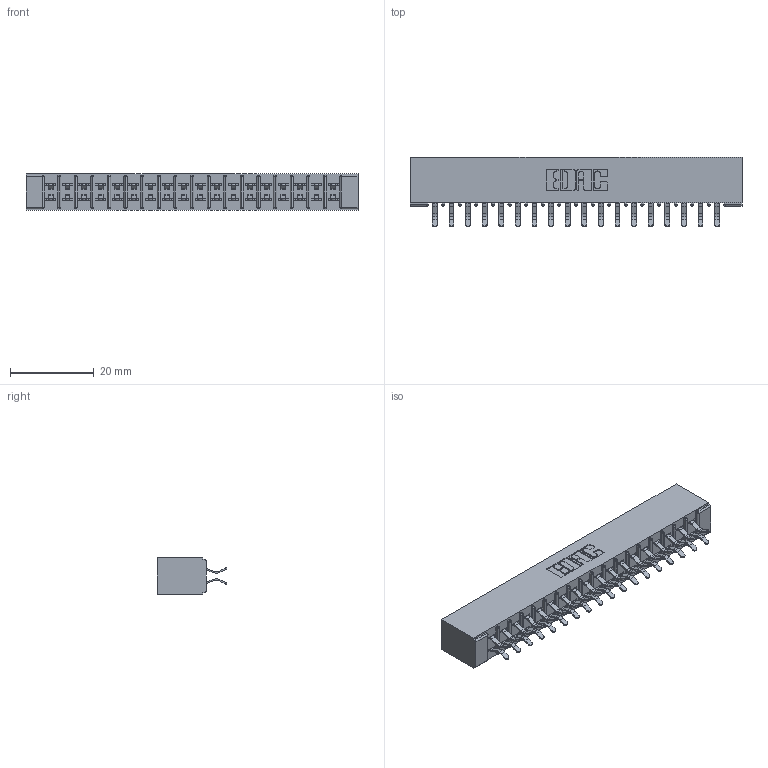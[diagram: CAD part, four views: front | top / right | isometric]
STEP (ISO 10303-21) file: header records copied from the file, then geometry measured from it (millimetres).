
FILE_DESCRIPTION (( 'STEP AP203' ), '1' );
FILE_NAME ('355-036-556-501.STEP', '2019-09-11T10:01:03', ( '' ), ( '' ), 'SwSTEP 2.0', 'SolidWorks 2016', '' );
FILE_SCHEMA (( 'CONFIG_CONTROL_DESIGN' ));
Length unit declared in the file: inch
Products named in the file (3): 355-036-556-501; 305-290-001_556; 305 Part_No Mounting
Assembly tree (37 placements, depth 2):
  355-036-556-501
    305 Part_No Mounting
    305-290-001_556  x36
Bounding box: 79.2 x 16.64 x 8.71 mm (x, y, z)
Volume: 4904.7 mm3; surface area: 10172.5 mm2
Topology: 37 solids, 37 shells, 2124 faces, 6106 edges, 3972 vertices
Faces by surface type: plane 1180, cylinder 872, sphere 72
Entity records: 22355 total; most frequent: CARTESIAN_POINT 3700, ORIENTED_EDGE 3668, DIRECTION 3600, EDGE_CURVE 1834, VECTOR 1456, LINE 1456, VERTEX_POINT 1172, AXIS2_PLACEMENT_3D 1072
